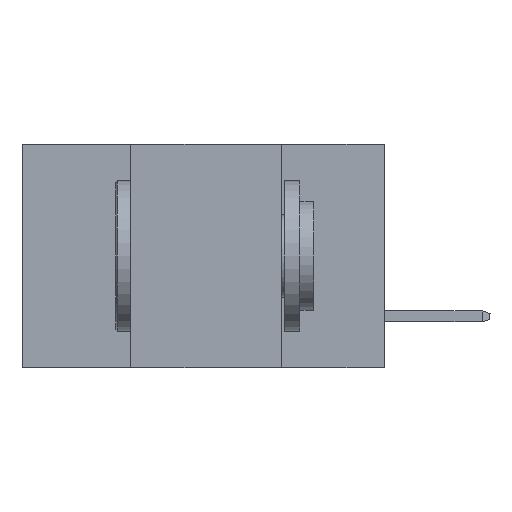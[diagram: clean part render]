
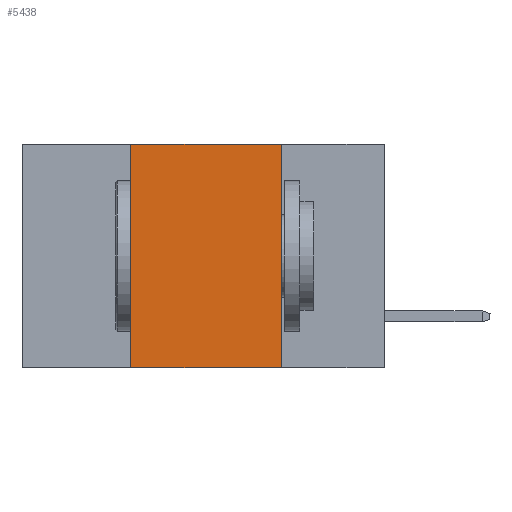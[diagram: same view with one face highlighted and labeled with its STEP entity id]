
A CAD part, left-side view. The second image highlights one B-rep face of the part: STEP entity #5438.
In plain terms, the highlighted planar face has unit normal (-1, 0, 0).
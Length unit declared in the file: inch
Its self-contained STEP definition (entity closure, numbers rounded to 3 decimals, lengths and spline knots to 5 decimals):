
#324 = EDGE_CURVE ( 'NONE', #14968, #1076, #12780, .T. ) ;
#485 = DIRECTION ( 'NONE',  ( 0., -1., 0. ) ) ;
#774 = VECTOR ( 'NONE', #12141, 39.37008 ) ;
#1076 = VERTEX_POINT ( 'NONE', #5551 ) ;
#1272 = VECTOR ( 'NONE', #4884, 39.37008 ) ;
#1522 = ORIENTED_EDGE ( 'NONE', *, *, #3764, .F. ) ;
#1591 = AXIS2_PLACEMENT_3D ( 'NONE', #6366, #10960, #8478 ) ;
#2785 = LINE ( 'NONE', #7306, #10098 ) ;
#2874 = CARTESIAN_POINT ( 'NONE',  ( 0., 0.42, -0.37 ) ) ;
#2899 = FACE_OUTER_BOUND ( 'NONE', #14313, .T. ) ;
#3764 = EDGE_CURVE ( 'NONE', #13901, #14968, #2785, .T. ) ;
#4080 = ORIENTED_EDGE ( 'NONE', *, *, #7311, .T. ) ;
#4132 = CARTESIAN_POINT ( 'NONE',  ( 0., 0.6, -0.37 ) ) ;
#4522 = EDGE_CURVE ( 'NONE', #12318, #13901, #6111, .T. ) ;
#4884 = DIRECTION ( 'NONE',  ( 0., 0., 1. ) ) ;
#5438 = ADVANCED_FACE ( 'NONE', ( #2899 ), #9610, .F. ) ;
#5539 = ORIENTED_EDGE ( 'NONE', *, *, #4522, .F. ) ;
#5551 = CARTESIAN_POINT ( 'NONE',  ( 0., 0.17, -0.37 ) ) ;
#6111 = LINE ( 'NONE', #2874, #1272 ) ;
#6366 = CARTESIAN_POINT ( 'NONE',  ( 0., 0.6, 0. ) ) ;
#6691 = CARTESIAN_POINT ( 'NONE',  ( 0., 0.42, -0.37 ) ) ;
#6700 = CARTESIAN_POINT ( 'NONE',  ( 0., 0.17, 0. ) ) ;
#6997 = CARTESIAN_POINT ( 'NONE',  ( 0., 0.17, -0.37 ) ) ;
#7306 = CARTESIAN_POINT ( 'NONE',  ( 0., 0.6, 0. ) ) ;
#7311 = EDGE_CURVE ( 'NONE', #12318, #1076, #10804, .T. ) ;
#8478 = DIRECTION ( 'NONE',  ( 0., 0., -1. ) ) ;
#9022 = ORIENTED_EDGE ( 'NONE', *, *, #324, .F. ) ;
#9050 = VECTOR ( 'NONE', #11610, 39.37008 ) ;
#9610 = PLANE ( 'NONE',  #1591 ) ;
#10098 = VECTOR ( 'NONE', #485, 39.37008 ) ;
#10804 = LINE ( 'NONE', #4132, #774 ) ;
#10960 = DIRECTION ( 'NONE',  ( 1., 0., 0. ) ) ;
#11610 = DIRECTION ( 'NONE',  ( 0., 0., -1. ) ) ;
#12141 = DIRECTION ( 'NONE',  ( 0., -1., 0. ) ) ;
#12217 = CARTESIAN_POINT ( 'NONE',  ( 0., 0.42, 0. ) ) ;
#12318 = VERTEX_POINT ( 'NONE', #6691 ) ;
#12780 = LINE ( 'NONE', #6997, #9050 ) ;
#13901 = VERTEX_POINT ( 'NONE', #12217 ) ;
#14313 = EDGE_LOOP ( 'NONE', ( #9022, #1522, #5539, #4080 ) ) ;
#14968 = VERTEX_POINT ( 'NONE', #6700 ) ;
